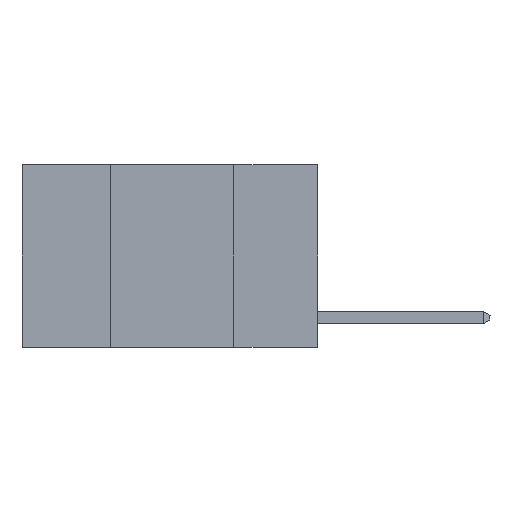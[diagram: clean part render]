
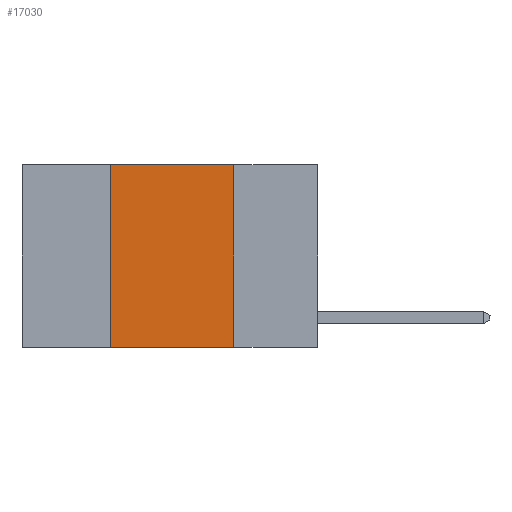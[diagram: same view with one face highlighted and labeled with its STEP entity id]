
A CAD part, left-side view. The second image highlights one B-rep face of the part: STEP entity #17030.
In plain terms, the highlighted planar face has unit normal (-1, 0, 0).
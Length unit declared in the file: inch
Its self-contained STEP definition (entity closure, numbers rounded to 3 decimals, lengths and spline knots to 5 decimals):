
#146 = VERTEX_POINT ( 'NONE', #13816 ) ;
#768 = AXIS2_PLACEMENT_3D ( 'NONE', #14173, #12748, #15656 ) ;
#1443 = CARTESIAN_POINT ( 'NONE',  ( 0., 0.6, -0.37 ) ) ;
#2160 = DIRECTION ( 'NONE',  ( 0., 0., -1. ) ) ;
#2491 = PLANE ( 'NONE',  #768 ) ;
#2929 = CARTESIAN_POINT ( 'NONE',  ( 0., 0.17, -0.37 ) ) ;
#4189 = ORIENTED_EDGE ( 'NONE', *, *, #4367, .T. ) ;
#4367 = EDGE_CURVE ( 'NONE', #12129, #8354, #14928, .T. ) ;
#4526 = VECTOR ( 'NONE', #2160, 39.37008 ) ;
#5757 = LINE ( 'NONE', #11936, #14710 ) ;
#6252 = ORIENTED_EDGE ( 'NONE', *, *, #17798, .F. ) ;
#7981 = CARTESIAN_POINT ( 'NONE',  ( 0., 0.6, 0. ) ) ;
#8249 = VERTEX_POINT ( 'NONE', #15166 ) ;
#8354 = VERTEX_POINT ( 'NONE', #2929 ) ;
#8379 = LINE ( 'NONE', #13832, #4526 ) ;
#8463 = ORIENTED_EDGE ( 'NONE', *, *, #14496, .F. ) ;
#9736 = CARTESIAN_POINT ( 'NONE',  ( 0., 0.42, -0.37 ) ) ;
#10305 = EDGE_LOOP ( 'NONE', ( #16511, #6252, #8463, #4189 ) ) ;
#11924 = LINE ( 'NONE', #7981, #16505 ) ;
#11936 = CARTESIAN_POINT ( 'NONE',  ( 0., 0.42, 0. ) ) ;
#12129 = VERTEX_POINT ( 'NONE', #9736 ) ;
#12748 = DIRECTION ( 'NONE',  ( 1., 0., 0. ) ) ;
#13816 = CARTESIAN_POINT ( 'NONE',  ( 0., 0.17, 0. ) ) ;
#13832 = CARTESIAN_POINT ( 'NONE',  ( 0., 0.17, 0. ) ) ;
#13891 = EDGE_CURVE ( 'NONE', #146, #8354, #8379, .T. ) ;
#14173 = CARTESIAN_POINT ( 'NONE',  ( 0., 0.6, 0. ) ) ;
#14441 = DIRECTION ( 'NONE',  ( 0., -1., 0. ) ) ;
#14496 = EDGE_CURVE ( 'NONE', #12129, #8249, #5757, .T. ) ;
#14710 = VECTOR ( 'NONE', #17678, 39.37008 ) ;
#14928 = LINE ( 'NONE', #1443, #15594 ) ;
#15166 = CARTESIAN_POINT ( 'NONE',  ( 0., 0.42, 0. ) ) ;
#15594 = VECTOR ( 'NONE', #14441, 39.37008 ) ;
#15656 = DIRECTION ( 'NONE',  ( 0., 0., -1. ) ) ;
#16505 = VECTOR ( 'NONE', #18226, 39.37008 ) ;
#16511 = ORIENTED_EDGE ( 'NONE', *, *, #13891, .F. ) ;
#17030 = ADVANCED_FACE ( 'NONE', ( #17205 ), #2491, .F. ) ;
#17205 = FACE_OUTER_BOUND ( 'NONE', #10305, .T. ) ;
#17678 = DIRECTION ( 'NONE',  ( 0., 0., 1. ) ) ;
#17798 = EDGE_CURVE ( 'NONE', #8249, #146, #11924, .T. ) ;
#18226 = DIRECTION ( 'NONE',  ( 0., -1., 0. ) ) ;
